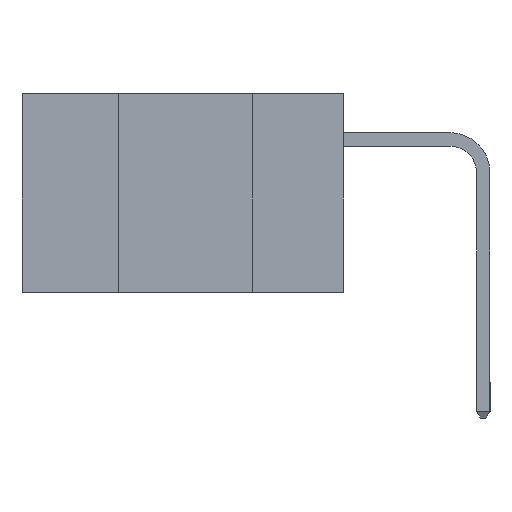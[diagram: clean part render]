
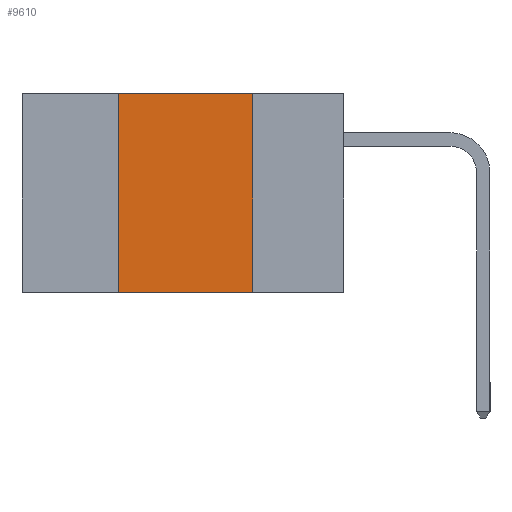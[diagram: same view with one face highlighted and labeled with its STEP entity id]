
A CAD part, left-side view. The second image highlights one B-rep face of the part: STEP entity #9610.
In plain terms, the highlighted planar face has unit normal (-1, 0, 0).
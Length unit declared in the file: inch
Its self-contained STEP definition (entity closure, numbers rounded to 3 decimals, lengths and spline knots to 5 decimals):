
#227 = EDGE_LOOP ( 'NONE', ( #9935, #3323, #6109, #7671 ) ) ;
#1065 = CARTESIAN_POINT ( 'NONE',  ( 0., 0.17, -0.37 ) ) ;
#1183 = CARTESIAN_POINT ( 'NONE',  ( 0., 0.42, 0. ) ) ;
#1405 = CARTESIAN_POINT ( 'NONE',  ( 0., 0.17, 0. ) ) ;
#1611 = VECTOR ( 'NONE', #2462, 39.37008 ) ;
#1784 = CARTESIAN_POINT ( 'NONE',  ( 0., 0.6, 0. ) ) ;
#2030 = LINE ( 'NONE', #9915, #2765 ) ;
#2462 = DIRECTION ( 'NONE',  ( 0., 0., 1. ) ) ;
#2484 = VECTOR ( 'NONE', #9987, 39.37008 ) ;
#2765 = VECTOR ( 'NONE', #8169, 39.37008 ) ;
#2782 = EDGE_CURVE ( 'NONE', #9487, #3477, #2030, .T. ) ;
#2847 = DIRECTION ( 'NONE',  ( 0., 0., -1. ) ) ;
#2975 = DIRECTION ( 'NONE',  ( 1., 0., 0. ) ) ;
#3323 = ORIENTED_EDGE ( 'NONE', *, *, #10814, .F. ) ;
#3477 = VERTEX_POINT ( 'NONE', #1065 ) ;
#3519 = CARTESIAN_POINT ( 'NONE',  ( 0., 0.6, 0. ) ) ;
#5371 = EDGE_CURVE ( 'NONE', #9487, #5524, #6888, .T. ) ;
#5524 = VERTEX_POINT ( 'NONE', #1183 ) ;
#6109 = ORIENTED_EDGE ( 'NONE', *, *, #5371, .F. ) ;
#6455 = LINE ( 'NONE', #3519, #11557 ) ;
#6831 = PLANE ( 'NONE',  #10721 ) ;
#6888 = LINE ( 'NONE', #8827, #1611 ) ;
#6896 = CARTESIAN_POINT ( 'NONE',  ( 0., 0.17, -0.37 ) ) ;
#7671 = ORIENTED_EDGE ( 'NONE', *, *, #2782, .T. ) ;
#7744 = CARTESIAN_POINT ( 'NONE',  ( 0., 0.42, -0.37 ) ) ;
#7926 = LINE ( 'NONE', #6896, #2484 ) ;
#7965 = VERTEX_POINT ( 'NONE', #1405 ) ;
#8169 = DIRECTION ( 'NONE',  ( 0., -1., 0. ) ) ;
#8716 = EDGE_CURVE ( 'NONE', #7965, #3477, #7926, .T. ) ;
#8827 = CARTESIAN_POINT ( 'NONE',  ( 0., 0.42, -0.37 ) ) ;
#9487 = VERTEX_POINT ( 'NONE', #7744 ) ;
#9610 = ADVANCED_FACE ( 'NONE', ( #9924 ), #6831, .F. ) ;
#9915 = CARTESIAN_POINT ( 'NONE',  ( 0., 0.6, -0.37 ) ) ;
#9924 = FACE_OUTER_BOUND ( 'NONE', #227, .T. ) ;
#9935 = ORIENTED_EDGE ( 'NONE', *, *, #8716, .F. ) ;
#9987 = DIRECTION ( 'NONE',  ( 0., 0., -1. ) ) ;
#10721 = AXIS2_PLACEMENT_3D ( 'NONE', #1784, #2975, #2847 ) ;
#10814 = EDGE_CURVE ( 'NONE', #5524, #7965, #6455, .T. ) ;
#11321 = DIRECTION ( 'NONE',  ( 0., -1., 0. ) ) ;
#11557 = VECTOR ( 'NONE', #11321, 39.37008 ) ;
